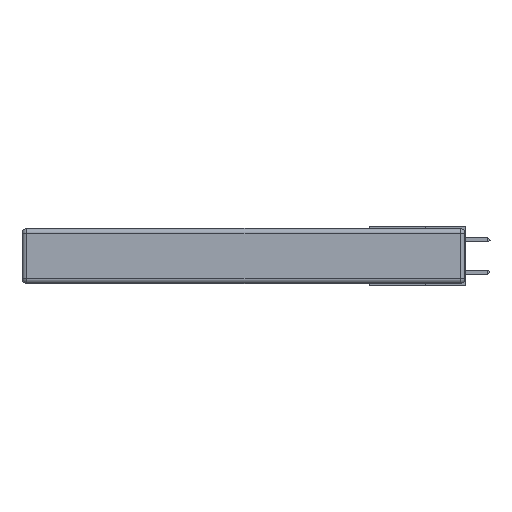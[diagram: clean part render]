
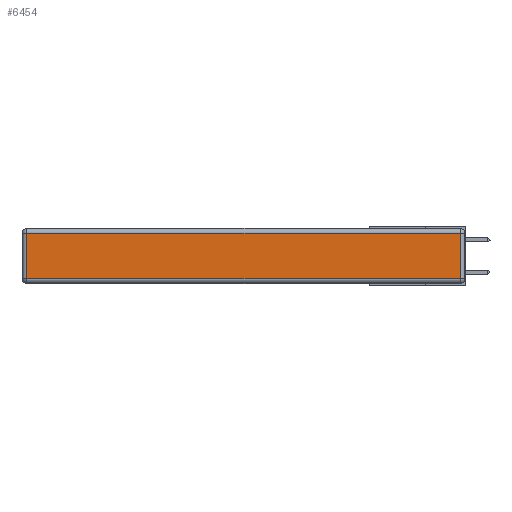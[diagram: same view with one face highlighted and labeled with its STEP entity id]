
A CAD part, left-side view. The second image highlights one B-rep face of the part: STEP entity #6454.
In plain terms, the highlighted planar face has unit normal (-1, 0, 0).
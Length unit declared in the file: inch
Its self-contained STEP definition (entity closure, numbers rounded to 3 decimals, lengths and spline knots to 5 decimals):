
#76 = ORIENTED_EDGE ( 'NONE', *, *, #3595, .T. ) ;
#290 = VECTOR ( 'NONE', #9365, 39.37008 ) ;
#485 = VECTOR ( 'NONE', #7812, 39.37008 ) ;
#960 = PLANE ( 'NONE',  #3404 ) ;
#1124 = LINE ( 'NONE', #16168, #10873 ) ;
#1723 = DIRECTION ( 'NONE',  ( 0., 0., 1. ) ) ;
#2037 = CARTESIAN_POINT ( 'NONE',  ( 0., 0.03, -0.313 ) ) ;
#3404 = AXIS2_PLACEMENT_3D ( 'NONE', #6224, #16965, #8927 ) ;
#3595 = EDGE_CURVE ( 'NONE', #6998, #6781, #10840, .T. ) ;
#3995 = VECTOR ( 'NONE', #1723, 39.37008 ) ;
#4007 = LINE ( 'NONE', #7966, #290 ) ;
#5074 = CARTESIAN_POINT ( 'NONE',  ( 0., 2.72, -0.03 ) ) ;
#6224 = CARTESIAN_POINT ( 'NONE',  ( 0., 0., -0.343 ) ) ;
#6343 = ORIENTED_EDGE ( 'NONE', *, *, #11058, .T. ) ;
#6454 = ADVANCED_FACE ( 'NONE', ( #11020 ), #960, .T. ) ;
#6680 = ORIENTED_EDGE ( 'NONE', *, *, #11035, .T. ) ;
#6781 = VERTEX_POINT ( 'NONE', #15888 ) ;
#6998 = VERTEX_POINT ( 'NONE', #2037 ) ;
#7812 = DIRECTION ( 'NONE',  ( 0., 1., 0. ) ) ;
#7966 = CARTESIAN_POINT ( 'NONE',  ( 0., 0., -0.313 ) ) ;
#8086 = DIRECTION ( 'NONE',  ( 0., 0., -1. ) ) ;
#8744 = CARTESIAN_POINT ( 'NONE',  ( 0., 2.72, -0.313 ) ) ;
#8927 = DIRECTION ( 'NONE',  ( 0., 0., 1. ) ) ;
#9266 = CARTESIAN_POINT ( 'NONE',  ( 0., 2.75, -0.03 ) ) ;
#9365 = DIRECTION ( 'NONE',  ( 0., -1., 0. ) ) ;
#9586 = CARTESIAN_POINT ( 'NONE',  ( 0., 0.03, -0.343 ) ) ;
#10541 = EDGE_LOOP ( 'NONE', ( #6343, #76, #12913, #6680 ) ) ;
#10820 = VERTEX_POINT ( 'NONE', #5074 ) ;
#10840 = LINE ( 'NONE', #9586, #3995 ) ;
#10873 = VECTOR ( 'NONE', #8086, 39.37008 ) ;
#11020 = FACE_OUTER_BOUND ( 'NONE', #10541, .T. ) ;
#11035 = EDGE_CURVE ( 'NONE', #10820, #14932, #1124, .T. ) ;
#11058 = EDGE_CURVE ( 'NONE', #14932, #6998, #4007, .T. ) ;
#12913 = ORIENTED_EDGE ( 'NONE', *, *, #17038, .T. ) ;
#13145 = LINE ( 'NONE', #9266, #485 ) ;
#14932 = VERTEX_POINT ( 'NONE', #8744 ) ;
#15888 = CARTESIAN_POINT ( 'NONE',  ( 0., 0.03, -0.03 ) ) ;
#16168 = CARTESIAN_POINT ( 'NONE',  ( 0., 2.72, -0.343 ) ) ;
#16965 = DIRECTION ( 'NONE',  ( -1., 0., 0. ) ) ;
#17038 = EDGE_CURVE ( 'NONE', #6781, #10820, #13145, .T. ) ;
